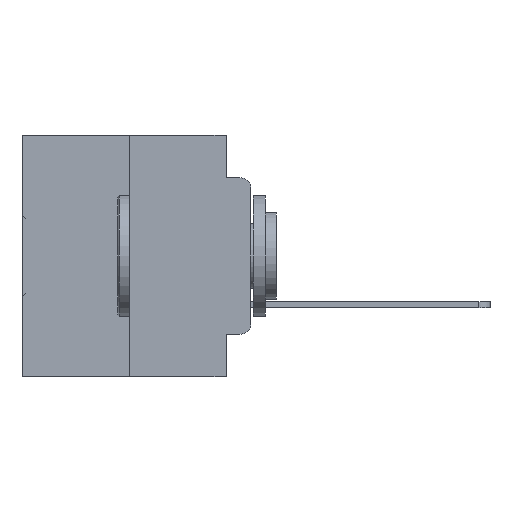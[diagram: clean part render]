
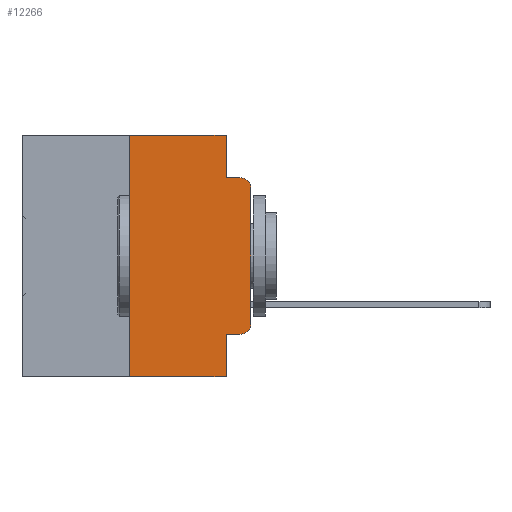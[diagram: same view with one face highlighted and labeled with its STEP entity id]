
A CAD part, left-side view. The second image highlights one B-rep face of the part: STEP entity #12266.
In plain terms, the highlighted planar face has unit normal (-1, 0, 0).
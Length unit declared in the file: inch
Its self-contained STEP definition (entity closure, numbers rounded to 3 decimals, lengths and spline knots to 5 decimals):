
#24 = LINE ( 'NONE', #21425, #27206 ) ;
#74 = CARTESIAN_POINT ( 'NONE',  ( 0., 0.02, -0.3915 ) ) ;
#304 = ORIENTED_EDGE ( 'NONE', *, *, #20766, .T. ) ;
#415 = VECTOR ( 'NONE', #28557, 39.37008 ) ;
#2134 = DIRECTION ( 'NONE',  ( 0., 0., 1. ) ) ;
#2210 = EDGE_CURVE ( 'NONE', #7862, #12715, #20745, .T. ) ;
#2422 = EDGE_CURVE ( 'NONE', #5556, #13459, #6705, .T. ) ;
#2628 = DIRECTION ( 'NONE',  ( 0., 0., -1. ) ) ;
#2885 = DIRECTION ( 'NONE',  ( 0., 0., -1. ) ) ;
#3000 = CARTESIAN_POINT ( 'NONE',  ( 0., 0., -0.1085 ) ) ;
#3092 = PLANE ( 'NONE',  #32165 ) ;
#3160 = VERTEX_POINT ( 'NONE', #14322 ) ;
#3455 = LINE ( 'NONE', #23208, #30421 ) ;
#4126 = CARTESIAN_POINT ( 'NONE',  ( 0., 0.473, -0.5 ) ) ;
#5272 = ORIENTED_EDGE ( 'NONE', *, *, #11710, .F. ) ;
#5430 = AXIS2_PLACEMENT_3D ( 'NONE', #34749, #19062, #2628 ) ;
#5556 = VERTEX_POINT ( 'NONE', #9330 ) ;
#5936 = DIRECTION ( 'NONE',  ( 0., 0., -1. ) ) ;
#5994 = CARTESIAN_POINT ( 'NONE',  ( 0., 0., -0.3915 ) ) ;
#6547 = VERTEX_POINT ( 'NONE', #18782 ) ;
#6636 = CARTESIAN_POINT ( 'NONE',  ( 0., 0.051, 0. ) ) ;
#6705 = CIRCLE ( 'NONE', #21442, 0.02 ) ;
#7519 = VECTOR ( 'NONE', #11689, 39.37008 ) ;
#7862 = VERTEX_POINT ( 'NONE', #25081 ) ;
#8021 = EDGE_CURVE ( 'NONE', #6547, #5556, #3455, .T. ) ;
#8908 = CARTESIAN_POINT ( 'NONE',  ( 0., 0.473, 0. ) ) ;
#9230 = LINE ( 'NONE', #8908, #7519 ) ;
#9330 = CARTESIAN_POINT ( 'NONE',  ( 0., 0.02, -0.4115 ) ) ;
#9402 = DIRECTION ( 'NONE',  ( 0., 0., -1. ) ) ;
#9870 = EDGE_CURVE ( 'NONE', #6547, #12715, #22151, .T. ) ;
#11240 = DIRECTION ( 'NONE',  ( 0., -1., 0. ) ) ;
#11298 = ORIENTED_EDGE ( 'NONE', *, *, #2422, .T. ) ;
#11358 = CARTESIAN_POINT ( 'NONE',  ( 0., 0.473, 0. ) ) ;
#11689 = DIRECTION ( 'NONE',  ( 0., -1., 0. ) ) ;
#11710 = EDGE_CURVE ( 'NONE', #7862, #3160, #21211, .T. ) ;
#12266 = ADVANCED_FACE ( 'NONE', ( #17854 ), #3092, .F. ) ;
#12596 = CARTESIAN_POINT ( 'NONE',  ( 0., 0.051, 0. ) ) ;
#12715 = VERTEX_POINT ( 'NONE', #15987 ) ;
#12854 = CIRCLE ( 'NONE', #5430, 0.02 ) ;
#13312 = CARTESIAN_POINT ( 'NONE',  ( 0., 0.051, -0.0885 ) ) ;
#13459 = VERTEX_POINT ( 'NONE', #5994 ) ;
#14322 = CARTESIAN_POINT ( 'NONE',  ( 0., 0.25, 0. ) ) ;
#15098 = DIRECTION ( 'NONE',  ( 0., -1., 0. ) ) ;
#15130 = LINE ( 'NONE', #12596, #415 ) ;
#15237 = ORIENTED_EDGE ( 'NONE', *, *, #18971, .F. ) ;
#15288 = DIRECTION ( 'NONE',  ( 0., -1., 0. ) ) ;
#15789 = ORIENTED_EDGE ( 'NONE', *, *, #29563, .T. ) ;
#15987 = CARTESIAN_POINT ( 'NONE',  ( 0., 0.051, -0.5 ) ) ;
#16092 = EDGE_CURVE ( 'NONE', #3160, #24304, #9230, .T. ) ;
#17191 = EDGE_CURVE ( 'NONE', #24304, #20332, #15130, .T. ) ;
#17223 = ORIENTED_EDGE ( 'NONE', *, *, #2210, .T. ) ;
#17854 = FACE_OUTER_BOUND ( 'NONE', #19786, .T. ) ;
#17883 = ORIENTED_EDGE ( 'NONE', *, *, #8021, .T. ) ;
#18588 = CARTESIAN_POINT ( 'NONE',  ( 0., 0.25, 0. ) ) ;
#18613 = VERTEX_POINT ( 'NONE', #33654 ) ;
#18782 = CARTESIAN_POINT ( 'NONE',  ( 0., 0.051, -0.4115 ) ) ;
#18971 = EDGE_CURVE ( 'NONE', #20332, #18613, #19612, .T. ) ;
#19062 = DIRECTION ( 'NONE',  ( -1., 0., 0. ) ) ;
#19326 = DIRECTION ( 'NONE',  ( -1., 0., 0. ) ) ;
#19612 = LINE ( 'NONE', #32476, #25802 ) ;
#19786 = EDGE_LOOP ( 'NONE', ( #15789, #304, #15237, #29243, #24053, #5272, #17223, #32080, #17883, #11298 ) ) ;
#20332 = VERTEX_POINT ( 'NONE', #13312 ) ;
#20745 = LINE ( 'NONE', #4126, #28564 ) ;
#20766 = EDGE_CURVE ( 'NONE', #22168, #18613, #12854, .T. ) ;
#21211 = LINE ( 'NONE', #18588, #29031 ) ;
#21425 = CARTESIAN_POINT ( 'NONE',  ( 0., 0., 0. ) ) ;
#21442 = AXIS2_PLACEMENT_3D ( 'NONE', #74, #19326, #2885 ) ;
#22151 = LINE ( 'NONE', #6636, #28357 ) ;
#22168 = VERTEX_POINT ( 'NONE', #3000 ) ;
#22169 = DIRECTION ( 'NONE',  ( 1., 0., 0. ) ) ;
#23208 = CARTESIAN_POINT ( 'NONE',  ( 0., 0.051, -0.4115 ) ) ;
#24053 = ORIENTED_EDGE ( 'NONE', *, *, #16092, .F. ) ;
#24072 = DIRECTION ( 'NONE',  ( 0., 0., 1. ) ) ;
#24304 = VERTEX_POINT ( 'NONE', #33304 ) ;
#25081 = CARTESIAN_POINT ( 'NONE',  ( 0., 0.25, -0.5 ) ) ;
#25802 = VECTOR ( 'NONE', #11240, 39.37008 ) ;
#27206 = VECTOR ( 'NONE', #24072, 39.37008 ) ;
#28357 = VECTOR ( 'NONE', #9402, 39.37008 ) ;
#28557 = DIRECTION ( 'NONE',  ( 0., 0., -1. ) ) ;
#28564 = VECTOR ( 'NONE', #15098, 39.37008 ) ;
#29031 = VECTOR ( 'NONE', #2134, 39.37008 ) ;
#29243 = ORIENTED_EDGE ( 'NONE', *, *, #17191, .F. ) ;
#29563 = EDGE_CURVE ( 'NONE', #13459, #22168, #24, .T. ) ;
#30421 = VECTOR ( 'NONE', #15288, 39.37008 ) ;
#32080 = ORIENTED_EDGE ( 'NONE', *, *, #9870, .F. ) ;
#32165 = AXIS2_PLACEMENT_3D ( 'NONE', #11358, #22169, #5936 ) ;
#32476 = CARTESIAN_POINT ( 'NONE',  ( 0., 0.051, -0.0885 ) ) ;
#33304 = CARTESIAN_POINT ( 'NONE',  ( 0., 0.051, 0. ) ) ;
#33654 = CARTESIAN_POINT ( 'NONE',  ( 0., 0.02, -0.0885 ) ) ;
#34749 = CARTESIAN_POINT ( 'NONE',  ( 0., 0.02, -0.1085 ) ) ;
